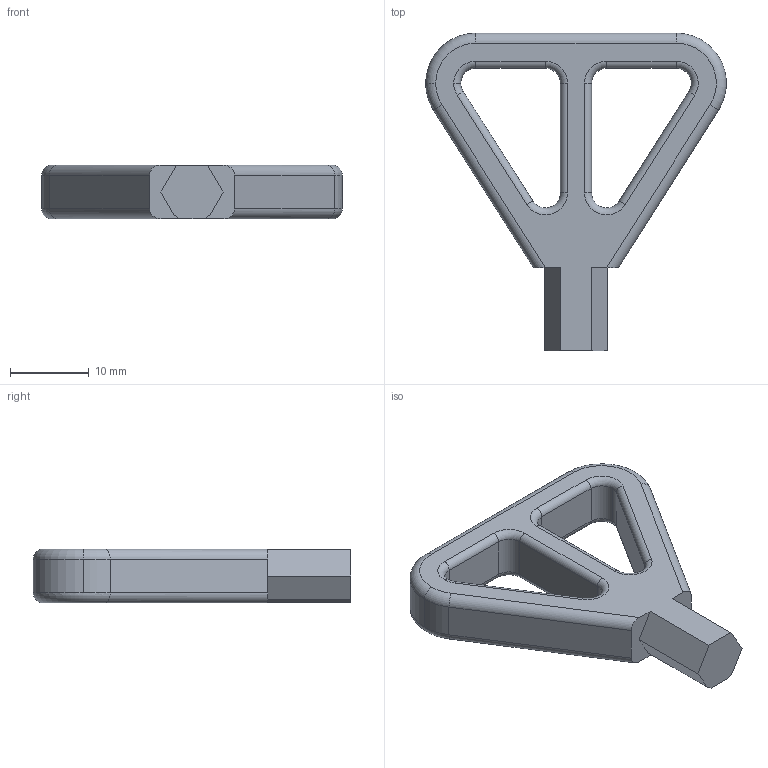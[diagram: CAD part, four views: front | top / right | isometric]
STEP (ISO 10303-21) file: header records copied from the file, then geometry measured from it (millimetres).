
FILE_DESCRIPTION (( 'STEP AP203' ), '1' );
FILE_NAME ('AF-HF-BT-PRT-001-STEP.STEP', '2020-10-04T16:20:20', ( '' ), ( '' ), 'SwSTEP 2.0', 'SolidWorks 2018', '' );
FILE_SCHEMA (( 'CONFIG_CONTROL_DESIGN' ));
Length unit declared in the file: inch
Products named in the file (1): AF-HF-BT-PRT-001-STEP
Bounding box: 38.1 x 40.26 x 6.83 mm (x, y, z)
Volume: 3912.9 mm3; surface area: 2565.6 mm2
Topology: 1 solids, 1 shells, 68 faces, 164 edges, 98 vertices
Faces by surface type: cylinder 28, torus 20, plane 20
Entity records: 2061 total; most frequent: DIRECTION 376, CARTESIAN_POINT 343, ORIENTED_EDGE 328, EDGE_CURVE 164, AXIS2_PLACEMENT_3D 147, VERTEX_POINT 98, VECTOR 82, LINE 82
